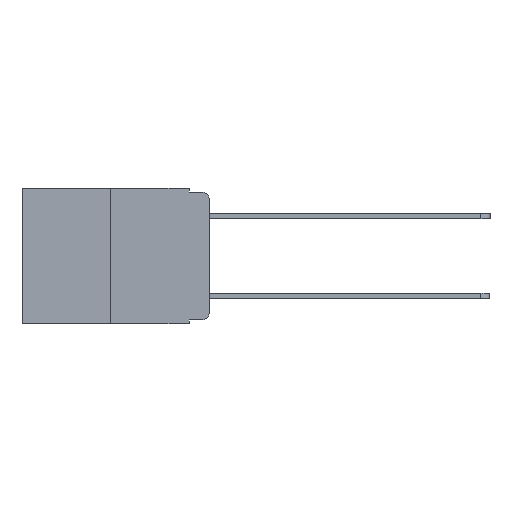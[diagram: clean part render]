
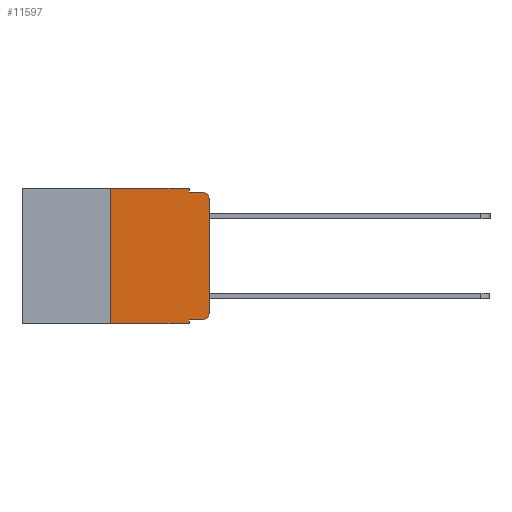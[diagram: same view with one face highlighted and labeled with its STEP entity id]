
A CAD part, left-side view. The second image highlights one B-rep face of the part: STEP entity #11597.
In plain terms, the highlighted planar face has unit normal (-1, 0, 0).
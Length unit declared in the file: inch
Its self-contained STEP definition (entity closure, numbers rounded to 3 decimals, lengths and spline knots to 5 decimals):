
#333 = VERTEX_POINT ( 'NONE', #6015 ) ;
#379 = DIRECTION ( 'NONE',  ( 0., 0., -1. ) ) ;
#475 = CIRCLE ( 'NONE', #10610, 0.02 ) ;
#557 = LINE ( 'NONE', #5750, #3658 ) ;
#656 = DIRECTION ( 'NONE',  ( -1., 0., 0. ) ) ;
#800 = VERTEX_POINT ( 'NONE', #7446 ) ;
#905 = DIRECTION ( 'NONE',  ( 0., -1., 0. ) ) ;
#914 = DIRECTION ( 'NONE',  ( 0., 0., -1. ) ) ;
#1014 = LINE ( 'NONE', #14414, #12993 ) ;
#1078 = VERTEX_POINT ( 'NONE', #8148 ) ;
#1233 = VECTOR ( 'NONE', #3767, 39.37008 ) ;
#2487 = VERTEX_POINT ( 'NONE', #14476 ) ;
#2558 = ORIENTED_EDGE ( 'NONE', *, *, #7029, .F. ) ;
#2567 = CARTESIAN_POINT ( 'NONE',  ( 0., 0.473, -0.343 ) ) ;
#2715 = AXIS2_PLACEMENT_3D ( 'NONE', #7090, #8200, #914 ) ;
#3114 = CARTESIAN_POINT ( 'NONE',  ( 0., 0.02, -0.01 ) ) ;
#3624 = LINE ( 'NONE', #5496, #6814 ) ;
#3658 = VECTOR ( 'NONE', #6916, 39.37008 ) ;
#3734 = ORIENTED_EDGE ( 'NONE', *, *, #6261, .F. ) ;
#3737 = CARTESIAN_POINT ( 'NONE',  ( 0., 0.02, -0.03 ) ) ;
#3767 = DIRECTION ( 'NONE',  ( 0., 0., -1. ) ) ;
#4159 = CARTESIAN_POINT ( 'NONE',  ( 0., 0.02, -0.333 ) ) ;
#4196 = ORIENTED_EDGE ( 'NONE', *, *, #4641, .T. ) ;
#4199 = VECTOR ( 'NONE', #905, 39.37008 ) ;
#4252 = VECTOR ( 'NONE', #379, 39.37008 ) ;
#4641 = EDGE_CURVE ( 'NONE', #10746, #2487, #6506, .T. ) ;
#4885 = ORIENTED_EDGE ( 'NONE', *, *, #5464, .T. ) ;
#4956 = DIRECTION ( 'NONE',  ( 0., 0., -1. ) ) ;
#5464 = EDGE_CURVE ( 'NONE', #9078, #10746, #14330, .T. ) ;
#5489 = CARTESIAN_POINT ( 'NONE',  ( 0., 0.25, -0.343 ) ) ;
#5496 = CARTESIAN_POINT ( 'NONE',  ( 0., 0., 0. ) ) ;
#5744 = VERTEX_POINT ( 'NONE', #10243 ) ;
#5750 = CARTESIAN_POINT ( 'NONE',  ( 0., 0.25, 0. ) ) ;
#6015 = CARTESIAN_POINT ( 'NONE',  ( 0., 0., -0.03 ) ) ;
#6190 = CARTESIAN_POINT ( 'NONE',  ( 0., 0.051, 0. ) ) ;
#6261 = EDGE_CURVE ( 'NONE', #9078, #5744, #13170, .T. ) ;
#6262 = LINE ( 'NONE', #2567, #11775 ) ;
#6301 = CARTESIAN_POINT ( 'NONE',  ( 0., 0.051, -0.333 ) ) ;
#6506 = CIRCLE ( 'NONE', #10920, 0.02 ) ;
#6814 = VECTOR ( 'NONE', #14273, 39.37008 ) ;
#6916 = DIRECTION ( 'NONE',  ( 0., 0., 1. ) ) ;
#6947 = EDGE_CURVE ( 'NONE', #12516, #1078, #1014, .T. ) ;
#7029 = EDGE_CURVE ( 'NONE', #14655, #12516, #557, .T. ) ;
#7090 = CARTESIAN_POINT ( 'NONE',  ( 0., 0.473, 0. ) ) ;
#7240 = ORIENTED_EDGE ( 'NONE', *, *, #11158, .T. ) ;
#7254 = EDGE_LOOP ( 'NONE', ( #8688, #13950, #12279, #8036, #9288, #2558, #7240, #3734, #4885, #4196 ) ) ;
#7446 = CARTESIAN_POINT ( 'NONE',  ( 0., 0.051, -0.01 ) ) ;
#7680 = LINE ( 'NONE', #14665, #4199 ) ;
#7773 = EDGE_CURVE ( 'NONE', #1078, #800, #10943, .T. ) ;
#8001 = CARTESIAN_POINT ( 'NONE',  ( 0., 0.02, -0.313 ) ) ;
#8036 = ORIENTED_EDGE ( 'NONE', *, *, #7773, .F. ) ;
#8148 = CARTESIAN_POINT ( 'NONE',  ( 0., 0.051, 0. ) ) ;
#8200 = DIRECTION ( 'NONE',  ( 1., 0., 0. ) ) ;
#8513 = EDGE_CURVE ( 'NONE', #800, #14680, #7680, .T. ) ;
#8688 = ORIENTED_EDGE ( 'NONE', *, *, #9994, .T. ) ;
#9062 = DIRECTION ( 'NONE',  ( 0., -1., 0. ) ) ;
#9078 = VERTEX_POINT ( 'NONE', #13259 ) ;
#9126 = DIRECTION ( 'NONE',  ( 0., 0., -1. ) ) ;
#9271 = EDGE_CURVE ( 'NONE', #333, #14680, #475, .T. ) ;
#9288 = ORIENTED_EDGE ( 'NONE', *, *, #6947, .F. ) ;
#9994 = EDGE_CURVE ( 'NONE', #2487, #333, #3624, .T. ) ;
#10243 = CARTESIAN_POINT ( 'NONE',  ( 0., 0.051, -0.343 ) ) ;
#10610 = AXIS2_PLACEMENT_3D ( 'NONE', #3737, #11653, #4956 ) ;
#10746 = VERTEX_POINT ( 'NONE', #4159 ) ;
#10920 = AXIS2_PLACEMENT_3D ( 'NONE', #8001, #656, #9126 ) ;
#10943 = LINE ( 'NONE', #6190, #1233 ) ;
#11158 = EDGE_CURVE ( 'NONE', #14655, #5744, #6262, .T. ) ;
#11597 = ADVANCED_FACE ( 'NONE', ( #13442 ), #14672, .F. ) ;
#11653 = DIRECTION ( 'NONE',  ( -1., 0., 0. ) ) ;
#11775 = VECTOR ( 'NONE', #12785, 39.37008 ) ;
#11830 = DIRECTION ( 'NONE',  ( 0., -1., 0. ) ) ;
#12279 = ORIENTED_EDGE ( 'NONE', *, *, #8513, .F. ) ;
#12516 = VERTEX_POINT ( 'NONE', #12943 ) ;
#12785 = DIRECTION ( 'NONE',  ( 0., -1., 0. ) ) ;
#12943 = CARTESIAN_POINT ( 'NONE',  ( 0., 0.25, 0. ) ) ;
#12993 = VECTOR ( 'NONE', #9062, 39.37008 ) ;
#13170 = LINE ( 'NONE', #13274, #4252 ) ;
#13259 = CARTESIAN_POINT ( 'NONE',  ( 0., 0.051, -0.333 ) ) ;
#13274 = CARTESIAN_POINT ( 'NONE',  ( 0., 0.051, 0. ) ) ;
#13442 = FACE_OUTER_BOUND ( 'NONE', #7254, .T. ) ;
#13950 = ORIENTED_EDGE ( 'NONE', *, *, #9271, .T. ) ;
#14011 = VECTOR ( 'NONE', #11830, 39.37008 ) ;
#14273 = DIRECTION ( 'NONE',  ( 0., 0., 1. ) ) ;
#14330 = LINE ( 'NONE', #6301, #14011 ) ;
#14414 = CARTESIAN_POINT ( 'NONE',  ( 0., 0.473, 0. ) ) ;
#14476 = CARTESIAN_POINT ( 'NONE',  ( 0., 0., -0.313 ) ) ;
#14655 = VERTEX_POINT ( 'NONE', #5489 ) ;
#14665 = CARTESIAN_POINT ( 'NONE',  ( 0., 0.051, -0.01 ) ) ;
#14672 = PLANE ( 'NONE',  #2715 ) ;
#14680 = VERTEX_POINT ( 'NONE', #3114 ) ;
